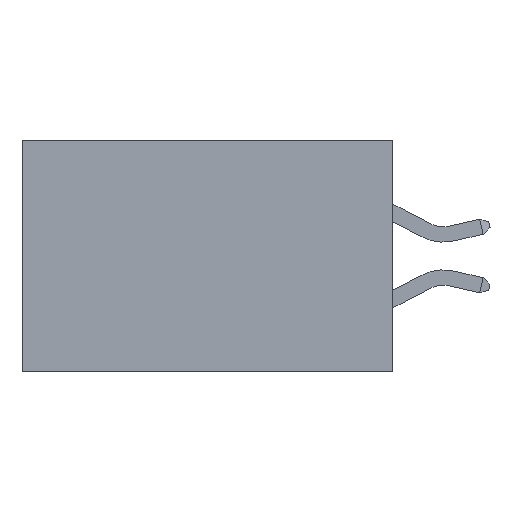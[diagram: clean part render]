
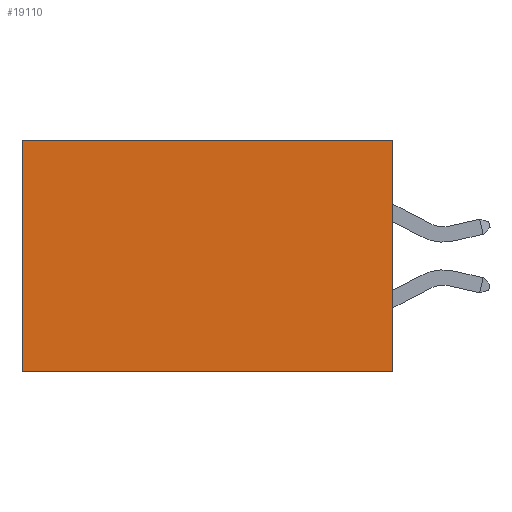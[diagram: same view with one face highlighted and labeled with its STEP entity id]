
A CAD part, left-side view. The second image highlights one B-rep face of the part: STEP entity #19110.
In plain terms, the highlighted planar face has unit normal (-1, 0, 0).
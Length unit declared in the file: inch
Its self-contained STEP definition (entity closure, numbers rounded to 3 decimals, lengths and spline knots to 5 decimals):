
#922 = ORIENTED_EDGE ( 'NONE', *, *, #1559, .F. ) ;
#1559 = EDGE_CURVE ( 'NONE', #15868, #9820, #7732, .T. ) ;
#1673 = LINE ( 'NONE', #17194, #10647 ) ;
#1810 = EDGE_CURVE ( 'NONE', #9820, #9193, #1673, .T. ) ;
#2169 = DIRECTION ( 'NONE',  ( 0., 0., -1. ) ) ;
#2531 = DIRECTION ( 'NONE',  ( 1., 0., 0. ) ) ;
#3284 = ORIENTED_EDGE ( 'NONE', *, *, #7531, .T. ) ;
#3445 = CARTESIAN_POINT ( 'NONE',  ( 0.2875, 0., 0. ) ) ;
#4318 = ORIENTED_EDGE ( 'NONE', *, *, #1810, .F. ) ;
#4371 = CARTESIAN_POINT ( 'NONE',  ( 0.2875, 0.6, -0.375 ) ) ;
#5905 = CARTESIAN_POINT ( 'NONE',  ( 0.2875, 0., -0.375 ) ) ;
#7220 = FACE_OUTER_BOUND ( 'NONE', #16859, .T. ) ;
#7531 = EDGE_CURVE ( 'NONE', #15868, #16163, #15172, .T. ) ;
#7700 = CARTESIAN_POINT ( 'NONE',  ( 0.2875, 0., -0.375 ) ) ;
#7732 = LINE ( 'NONE', #15055, #20715 ) ;
#8141 = DIRECTION ( 'NONE',  ( 0., 1., 0. ) ) ;
#8414 = CARTESIAN_POINT ( 'NONE',  ( 0.2875, 0.6, 0. ) ) ;
#9193 = VERTEX_POINT ( 'NONE', #4371 ) ;
#9439 = ORIENTED_EDGE ( 'NONE', *, *, #11649, .T. ) ;
#9820 = VERTEX_POINT ( 'NONE', #7700 ) ;
#10206 = AXIS2_PLACEMENT_3D ( 'NONE', #5905, #2531, #19555 ) ;
#10280 = DIRECTION ( 'NONE',  ( 0., 1., 0. ) ) ;
#10647 = VECTOR ( 'NONE', #10280, 39.37008 ) ;
#10773 = CARTESIAN_POINT ( 'NONE',  ( 0.2875, 0.6, -0.375 ) ) ;
#11649 = EDGE_CURVE ( 'NONE', #16163, #9193, #18163, .T. ) ;
#14633 = VECTOR ( 'NONE', #8141, 39.37008 ) ;
#15055 = CARTESIAN_POINT ( 'NONE',  ( 0.2875, 0., -0.375 ) ) ;
#15172 = LINE ( 'NONE', #3445, #14633 ) ;
#15637 = CARTESIAN_POINT ( 'NONE',  ( 0.2875, 0., 0. ) ) ;
#15868 = VERTEX_POINT ( 'NONE', #15637 ) ;
#16163 = VERTEX_POINT ( 'NONE', #8414 ) ;
#16859 = EDGE_LOOP ( 'NONE', ( #9439, #4318, #922, #3284 ) ) ;
#17194 = CARTESIAN_POINT ( 'NONE',  ( 0.2875, 0., -0.375 ) ) ;
#17846 = PLANE ( 'NONE',  #10206 ) ;
#18045 = DIRECTION ( 'NONE',  ( 0., 0., -1. ) ) ;
#18163 = LINE ( 'NONE', #10773, #19773 ) ;
#19110 = ADVANCED_FACE ( 'NONE', ( #7220 ), #17846, .F. ) ;
#19555 = DIRECTION ( 'NONE',  ( 0., 0., -1. ) ) ;
#19773 = VECTOR ( 'NONE', #2169, 39.37008 ) ;
#20715 = VECTOR ( 'NONE', #18045, 39.37008 ) ;
